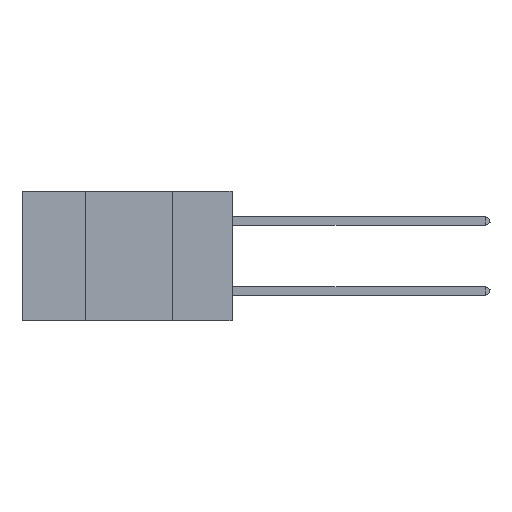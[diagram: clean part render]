
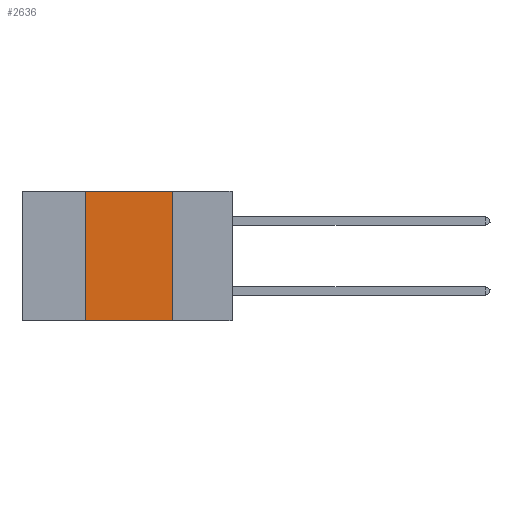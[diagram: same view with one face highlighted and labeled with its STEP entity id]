
A CAD part, left-side view. The second image highlights one B-rep face of the part: STEP entity #2636.
In plain terms, the highlighted planar face has unit normal (-1, 0, 0).
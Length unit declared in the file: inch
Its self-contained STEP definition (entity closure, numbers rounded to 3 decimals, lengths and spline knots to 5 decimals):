
#646 = VECTOR ( 'NONE', #30622, 39.37008 ) ;
#1832 = VECTOR ( 'NONE', #7519, 39.37008 ) ;
#2212 = EDGE_CURVE ( 'NONE', #21985, #2297, #20016, .T. ) ;
#2297 = VERTEX_POINT ( 'NONE', #30908 ) ;
#2470 = DIRECTION ( 'NONE',  ( 1., 0., 0. ) ) ;
#2636 = ADVANCED_FACE ( 'NONE', ( #11532 ), #35267, .F. ) ;
#3981 = VECTOR ( 'NONE', #12748, 39.37008 ) ;
#4417 = CARTESIAN_POINT ( 'NONE',  ( 0., 0.42, 0. ) ) ;
#5059 = LINE ( 'NONE', #14286, #27984 ) ;
#7519 = DIRECTION ( 'NONE',  ( 0., 0., 1. ) ) ;
#10249 = ORIENTED_EDGE ( 'NONE', *, *, #29276, .T. ) ;
#11458 = VERTEX_POINT ( 'NONE', #35750 ) ;
#11532 = FACE_OUTER_BOUND ( 'NONE', #35845, .T. ) ;
#12748 = DIRECTION ( 'NONE',  ( 0., 0., -1. ) ) ;
#14286 = CARTESIAN_POINT ( 'NONE',  ( 0., 0.6, -0.37 ) ) ;
#16750 = LINE ( 'NONE', #18737, #646 ) ;
#17271 = DIRECTION ( 'NONE',  ( 0., -1., 0. ) ) ;
#17512 = ORIENTED_EDGE ( 'NONE', *, *, #2212, .F. ) ;
#17582 = VERTEX_POINT ( 'NONE', #32746 ) ;
#18737 = CARTESIAN_POINT ( 'NONE',  ( 0., 0.6, 0. ) ) ;
#20016 = LINE ( 'NONE', #24560, #3981 ) ;
#21985 = VERTEX_POINT ( 'NONE', #26534 ) ;
#23311 = AXIS2_PLACEMENT_3D ( 'NONE', #26337, #2470, #23490 ) ;
#23490 = DIRECTION ( 'NONE',  ( 0., 0., -1. ) ) ;
#24540 = ORIENTED_EDGE ( 'NONE', *, *, #33746, .F. ) ;
#24560 = CARTESIAN_POINT ( 'NONE',  ( 0., 0.17, 0. ) ) ;
#25775 = LINE ( 'NONE', #4417, #1832 ) ;
#26337 = CARTESIAN_POINT ( 'NONE',  ( 0., 0.6, 0. ) ) ;
#26534 = CARTESIAN_POINT ( 'NONE',  ( 0., 0.17, 0. ) ) ;
#27607 = ORIENTED_EDGE ( 'NONE', *, *, #30935, .F. ) ;
#27984 = VECTOR ( 'NONE', #17271, 39.37008 ) ;
#29276 = EDGE_CURVE ( 'NONE', #17582, #2297, #5059, .T. ) ;
#30622 = DIRECTION ( 'NONE',  ( 0., -1., 0. ) ) ;
#30908 = CARTESIAN_POINT ( 'NONE',  ( 0., 0.17, -0.37 ) ) ;
#30935 = EDGE_CURVE ( 'NONE', #11458, #21985, #16750, .T. ) ;
#32746 = CARTESIAN_POINT ( 'NONE',  ( 0., 0.42, -0.37 ) ) ;
#33746 = EDGE_CURVE ( 'NONE', #17582, #11458, #25775, .T. ) ;
#35267 = PLANE ( 'NONE',  #23311 ) ;
#35750 = CARTESIAN_POINT ( 'NONE',  ( 0., 0.42, 0. ) ) ;
#35845 = EDGE_LOOP ( 'NONE', ( #17512, #27607, #24540, #10249 ) ) ;
